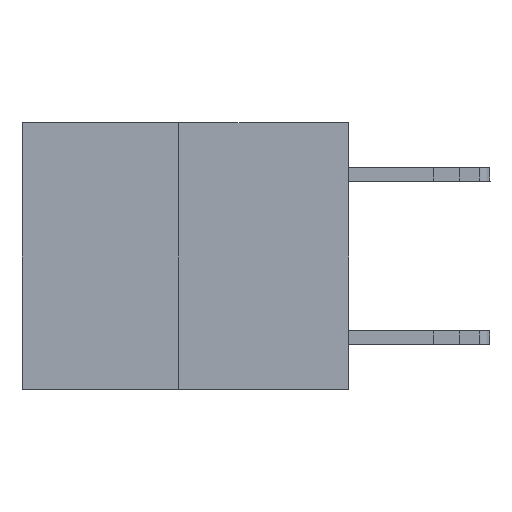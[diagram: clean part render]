
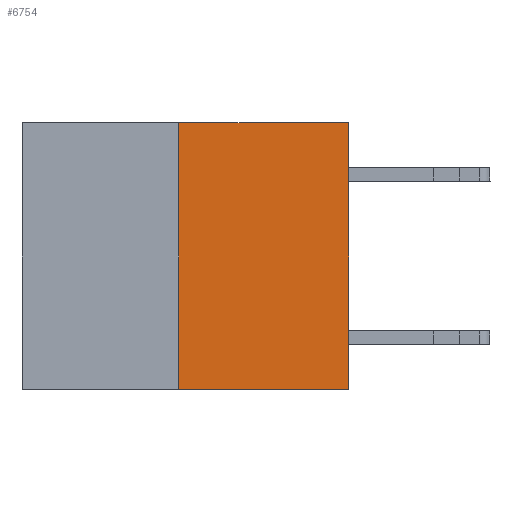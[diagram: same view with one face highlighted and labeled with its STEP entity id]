
A CAD part, left-side view. The second image highlights one B-rep face of the part: STEP entity #6754.
In plain terms, the highlighted planar face has unit normal (-1, 0, 0).
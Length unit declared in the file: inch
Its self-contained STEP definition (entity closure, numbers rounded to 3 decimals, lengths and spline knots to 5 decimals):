
#344 = CARTESIAN_POINT ( 'NONE',  ( 0., 0.6, 0. ) ) ;
#773 = VECTOR ( 'NONE', #12950, 39.37008 ) ;
#1098 = ORIENTED_EDGE ( 'NONE', *, *, #22856, .T. ) ;
#1219 = CARTESIAN_POINT ( 'NONE',  ( 0., 0., 0. ) ) ;
#1303 = DIRECTION ( 'NONE',  ( 0., 0., 1. ) ) ;
#1655 = VECTOR ( 'NONE', #19571, 39.37008 ) ;
#3554 = ORIENTED_EDGE ( 'NONE', *, *, #25591, .F. ) ;
#4212 = AXIS2_PLACEMENT_3D ( 'NONE', #344, #10642, #22904 ) ;
#4686 = VECTOR ( 'NONE', #1303, 39.37008 ) ;
#6376 = VERTEX_POINT ( 'NONE', #12563 ) ;
#6754 = ADVANCED_FACE ( 'NONE', ( #19061 ), #8721, .F. ) ;
#6878 = CARTESIAN_POINT ( 'NONE',  ( 0., 0.6, -0.49 ) ) ;
#7041 = EDGE_LOOP ( 'NONE', ( #11458, #1098, #17881, #3554 ) ) ;
#8721 = PLANE ( 'NONE',  #4212 ) ;
#10642 = DIRECTION ( 'NONE',  ( 1., 0., 0. ) ) ;
#11284 = LINE ( 'NONE', #23871, #1655 ) ;
#11458 = ORIENTED_EDGE ( 'NONE', *, *, #18729, .F. ) ;
#11728 = LINE ( 'NONE', #1219, #4686 ) ;
#12563 = CARTESIAN_POINT ( 'NONE',  ( 0., 0.312, -0.49 ) ) ;
#12814 = CARTESIAN_POINT ( 'NONE',  ( 0., 0., 0. ) ) ;
#12950 = DIRECTION ( 'NONE',  ( 0., -1., 0. ) ) ;
#13397 = VERTEX_POINT ( 'NONE', #13451 ) ;
#13451 = CARTESIAN_POINT ( 'NONE',  ( 0., 0.312, 0. ) ) ;
#14638 = VERTEX_POINT ( 'NONE', #12814 ) ;
#16990 = CARTESIAN_POINT ( 'NONE',  ( 0., 0.6, 0. ) ) ;
#17881 = ORIENTED_EDGE ( 'NONE', *, *, #21996, .T. ) ;
#17977 = CARTESIAN_POINT ( 'NONE',  ( 0., 0., -0.49 ) ) ;
#18468 = LINE ( 'NONE', #6878, #773 ) ;
#18729 = EDGE_CURVE ( 'NONE', #6376, #13397, #11284, .T. ) ;
#19061 = FACE_OUTER_BOUND ( 'NONE', #7041, .T. ) ;
#19571 = DIRECTION ( 'NONE',  ( 0., 0., 1. ) ) ;
#20882 = DIRECTION ( 'NONE',  ( 0., -1., 0. ) ) ;
#21658 = VERTEX_POINT ( 'NONE', #17977 ) ;
#21996 = EDGE_CURVE ( 'NONE', #21658, #14638, #11728, .T. ) ;
#22856 = EDGE_CURVE ( 'NONE', #6376, #21658, #18468, .T. ) ;
#22859 = VECTOR ( 'NONE', #20882, 39.37008 ) ;
#22904 = DIRECTION ( 'NONE',  ( 0., 0., -1. ) ) ;
#23871 = CARTESIAN_POINT ( 'NONE',  ( 0., 0.312, -0.49 ) ) ;
#24154 = LINE ( 'NONE', #16990, #22859 ) ;
#25591 = EDGE_CURVE ( 'NONE', #13397, #14638, #24154, .T. ) ;
